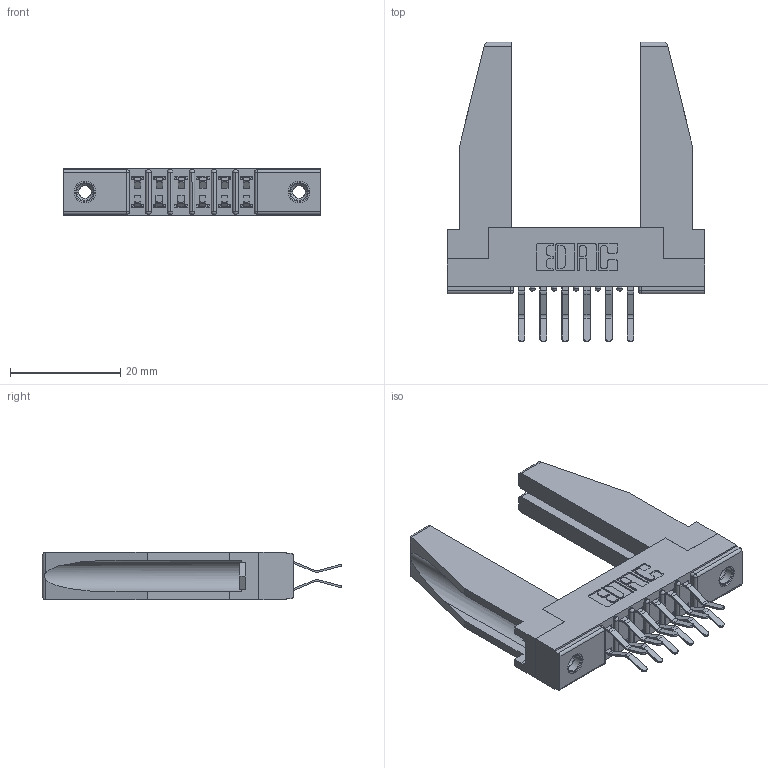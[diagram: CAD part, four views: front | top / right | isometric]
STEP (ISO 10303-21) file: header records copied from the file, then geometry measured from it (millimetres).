
FILE_DESCRIPTION (( 'STEP AP203' ), '1' );
FILE_NAME ('357-012-560-278.STEP', '2019-09-17T18:19:20', ( '' ), ( '' ), 'SwSTEP 2.0', 'SolidWorks 2016', '' );
FILE_SCHEMA (( 'CONFIG_CONTROL_DESIGN' ));
Length unit declared in the file: inch
Products named in the file (5): 345-250-001_345-250-001-102; 307-290-001_560; 307 Part_.156 Dia Mounting Holes; 307-220-078; 357-012-560-278
Assembly tree (17 placements, depth 2):
  357-012-560-278
    307 Part_.156 Dia Mounting Holes
    307-290-001_560  x12
    307-220-078  x2
    345-250-001_345-250-001-102  x2
Bounding box: 46.79 x 54.43 x 8.71 mm (x, y, z)
Volume: 7070.4 mm3; surface area: 8515.4 mm2
Topology: 17 solids, 17 shells, 855 faces, 2357 edges, 1526 vertices
Faces by surface type: plane 550, cylinder 275, sphere 14, cone 12, torus 4
Entity records: 12317 total; most frequent: CARTESIAN_POINT 2036, ORIENTED_EDGE 1972, DIRECTION 1964, EDGE_CURVE 986, LINE 744, VECTOR 744, VERTEX_POINT 640, AXIS2_PLACEMENT_3D 610
